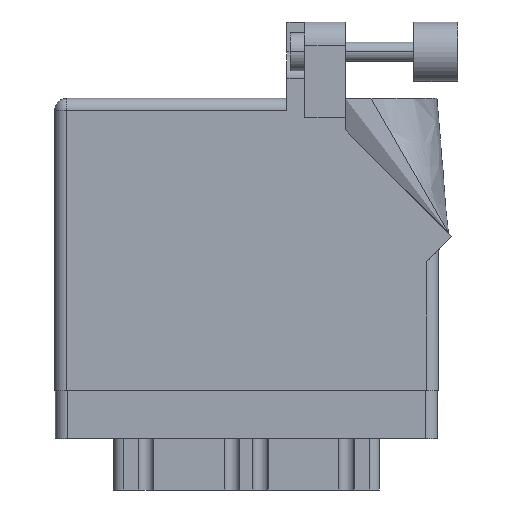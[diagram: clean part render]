
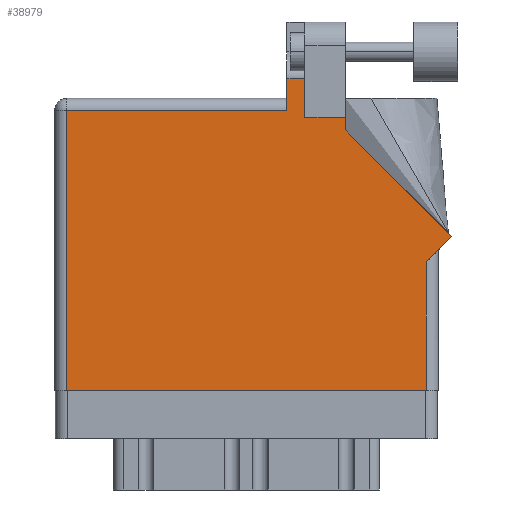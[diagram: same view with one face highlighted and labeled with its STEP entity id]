
A CAD part, front view. The second image highlights one B-rep face of the part: STEP entity #38979.
In plain terms, the highlighted face is planar.
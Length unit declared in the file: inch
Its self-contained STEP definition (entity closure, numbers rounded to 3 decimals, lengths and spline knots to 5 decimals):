
#32 = ORIENTED_EDGE ( 'NONE', *, *, #8942, .T. ) ;
#336 = CARTESIAN_POINT ( 'NONE',  ( 1.524, 1.43, 0. ) ) ;
#1288 = DIRECTION ( 'NONE',  ( 0., 1., 0. ) ) ;
#1882 = VERTEX_POINT ( 'NONE', #16018 ) ;
#3654 = CARTESIAN_POINT ( 'NONE',  ( 2.08071, 0.80771, 0. ) ) ;
#3865 = VECTOR ( 'NONE', #17499, 39.37008 ) ;
#3977 = VERTEX_POINT ( 'NONE', #27206 ) ;
#4223 = ORIENTED_EDGE ( 'NONE', *, *, #35668, .T. ) ;
#5249 = LINE ( 'NONE', #26387, #3865 ) ;
#5605 = ORIENTED_EDGE ( 'NONE', *, *, #30970, .T. ) ;
#5724 = VECTOR ( 'NONE', #1288, 39.37008 ) ;
#5999 = AXIS2_PLACEMENT_3D ( 'NONE', #10548, #13889, #37233 ) ;
#6206 = VECTOR ( 'NONE', #22170, 39.37008 ) ;
#6541 = ORIENTED_EDGE ( 'NONE', *, *, #27113, .T. ) ;
#6865 = VECTOR ( 'NONE', #21442, 39.37008 ) ;
#7092 = VECTOR ( 'NONE', #21846, 39.37008 ) ;
#8240 = VERTEX_POINT ( 'NONE', #20015 ) ;
#8293 = EDGE_CURVE ( 'NONE', #24620, #18932, #29703, .T. ) ;
#8359 = DIRECTION ( 'NONE',  ( 0., -1., 0. ) ) ;
#8633 = ORIENTED_EDGE ( 'NONE', *, *, #21370, .T. ) ;
#8942 = EDGE_CURVE ( 'NONE', #8240, #9744, #15597, .T. ) ;
#9248 = LINE ( 'NONE', #15562, #16901 ) ;
#9288 = ORIENTED_EDGE ( 'NONE', *, *, #28145, .T. ) ;
#9343 = VERTEX_POINT ( 'NONE', #18145 ) ;
#9466 = VECTOR ( 'NONE', #15013, 39.37008 ) ;
#9723 = LINE ( 'NONE', #37181, #6206 ) ;
#9744 = VERTEX_POINT ( 'NONE', #23231 ) ;
#10548 = CARTESIAN_POINT ( 'NONE',  ( 0., 1.53, 0. ) ) ;
#10600 = DIRECTION ( 'NONE',  ( -1., 0., 0. ) ) ;
#11917 = LINE ( 'NONE', #29920, #12676 ) ;
#12012 = VECTOR ( 'NONE', #10600, 39.37008 ) ;
#12676 = VECTOR ( 'NONE', #29716, 39.37008 ) ;
#13034 = ORIENTED_EDGE ( 'NONE', *, *, #23957, .T. ) ;
#13889 = DIRECTION ( 'NONE',  ( 0., 0., -1. ) ) ;
#14204 = ORIENTED_EDGE ( 'NONE', *, *, #8293, .T. ) ;
#14240 = CARTESIAN_POINT ( 'NONE',  ( 0.062, 1.468, 0. ) ) ;
#15013 = DIRECTION ( 'NONE',  ( 0., 1., 0. ) ) ;
#15562 = CARTESIAN_POINT ( 'NONE',  ( 2.01, 0.737, 0. ) ) ;
#15597 = LINE ( 'NONE', #17808, #9466 ) ;
#15955 = LINE ( 'NONE', #25433, #12012 ) ;
#16018 = CARTESIAN_POINT ( 'NONE',  ( 1.524, 1.36442, 0. ) ) ;
#16536 = DIRECTION ( 'NONE',  ( -1., 0., 0. ) ) ;
#16901 = VECTOR ( 'NONE', #30409, 39.37008 ) ;
#17499 = DIRECTION ( 'NONE',  ( -1., 0., 0. ) ) ;
#17562 = VERTEX_POINT ( 'NONE', #336 ) ;
#17808 = CARTESIAN_POINT ( 'NONE',  ( 1.948, 0.737, 0. ) ) ;
#18141 = ORIENTED_EDGE ( 'NONE', *, *, #35921, .T. ) ;
#18145 = CARTESIAN_POINT ( 'NONE',  ( 0.062, 0., 0. ) ) ;
#18496 = LINE ( 'NONE', #3654, #6865 ) ;
#18533 = CARTESIAN_POINT ( 'NONE',  ( 2.08071, 0.80771, 0. ) ) ;
#18932 = VERTEX_POINT ( 'NONE', #28954 ) ;
#19301 = CARTESIAN_POINT ( 'NONE',  ( 1.311, 1.43, 0. ) ) ;
#19462 = CARTESIAN_POINT ( 'NONE',  ( 0.062, 0., 0. ) ) ;
#19759 = ORIENTED_EDGE ( 'NONE', *, *, #26512, .T. ) ;
#20015 = CARTESIAN_POINT ( 'NONE',  ( 1.948, 0., 0. ) ) ;
#21266 = VERTEX_POINT ( 'NONE', #18533 ) ;
#21370 = EDGE_CURVE ( 'NONE', #3977, #24620, #15955, .T. ) ;
#21442 = DIRECTION ( 'NONE',  ( -0.707, 0.707, 0. ) ) ;
#21846 = DIRECTION ( 'NONE',  ( 0., -1., 0. ) ) ;
#22170 = DIRECTION ( 'NONE',  ( 1., 0., 0. ) ) ;
#22276 = CARTESIAN_POINT ( 'NONE',  ( 0., 1.468, 0. ) ) ;
#22418 = VERTEX_POINT ( 'NONE', #14240 ) ;
#22426 = CARTESIAN_POINT ( 'NONE',  ( 1.311, 1.43, 0. ) ) ;
#22488 = ORIENTED_EDGE ( 'NONE', *, *, #37021, .T. ) ;
#23231 = CARTESIAN_POINT ( 'NONE',  ( 1.948, 0.675, 0. ) ) ;
#23957 = EDGE_CURVE ( 'NONE', #18932, #22418, #28592, .T. ) ;
#24620 = VERTEX_POINT ( 'NONE', #29463 ) ;
#24800 = LINE ( 'NONE', #22426, #5724 ) ;
#25260 = VERTEX_POINT ( 'NONE', #19301 ) ;
#25433 = CARTESIAN_POINT ( 'NONE',  ( 1.64177, 1.6315, 0. ) ) ;
#25562 = PLANE ( 'NONE',  #5999 ) ;
#26387 = CARTESIAN_POINT ( 'NONE',  ( 1.524, 1.43, 0. ) ) ;
#26512 = EDGE_CURVE ( 'NONE', #9744, #21266, #9248, .T. ) ;
#27113 = EDGE_CURVE ( 'NONE', #9343, #8240, #9723, .T. ) ;
#27206 = CARTESIAN_POINT ( 'NONE',  ( 1.311, 1.6315, 0. ) ) ;
#28145 = EDGE_CURVE ( 'NONE', #17562, #25260, #5249, .T. ) ;
#28592 = LINE ( 'NONE', #22276, #30479 ) ;
#28753 = LINE ( 'NONE', #19462, #7092 ) ;
#28954 = CARTESIAN_POINT ( 'NONE',  ( 1.217, 1.468, 0. ) ) ;
#29463 = CARTESIAN_POINT ( 'NONE',  ( 1.217, 1.6315, 0. ) ) ;
#29703 = LINE ( 'NONE', #35637, #38477 ) ;
#29716 = DIRECTION ( 'NONE',  ( 0., 1., 0. ) ) ;
#29920 = CARTESIAN_POINT ( 'NONE',  ( 1.524, 1.36442, 0. ) ) ;
#30409 = DIRECTION ( 'NONE',  ( 0.707, 0.707, 0. ) ) ;
#30479 = VECTOR ( 'NONE', #16536, 39.37008 ) ;
#30970 = EDGE_CURVE ( 'NONE', #21266, #1882, #18496, .T. ) ;
#34668 = FACE_OUTER_BOUND ( 'NONE', #35031, .T. ) ;
#35031 = EDGE_LOOP ( 'NONE', ( #4223, #8633, #14204, #13034, #22488, #6541, #32, #19759, #5605, #18141, #9288 ) ) ;
#35637 = CARTESIAN_POINT ( 'NONE',  ( 1.217, 1.53, 0. ) ) ;
#35668 = EDGE_CURVE ( 'NONE', #25260, #3977, #24800, .T. ) ;
#35921 = EDGE_CURVE ( 'NONE', #1882, #17562, #11917, .T. ) ;
#37021 = EDGE_CURVE ( 'NONE', #22418, #9343, #28753, .T. ) ;
#37181 = CARTESIAN_POINT ( 'NONE',  ( 0., 0., 0. ) ) ;
#37233 = DIRECTION ( 'NONE',  ( -1., 0., 0. ) ) ;
#38477 = VECTOR ( 'NONE', #8359, 39.37008 ) ;
#38979 = ADVANCED_FACE ( 'NONE', ( #34668 ), #25562, .F. ) ;
